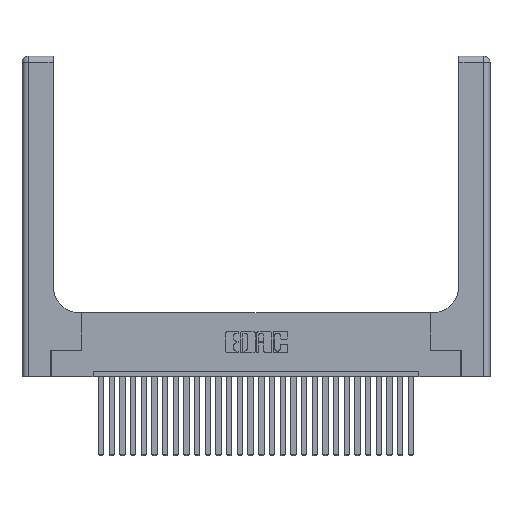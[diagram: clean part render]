
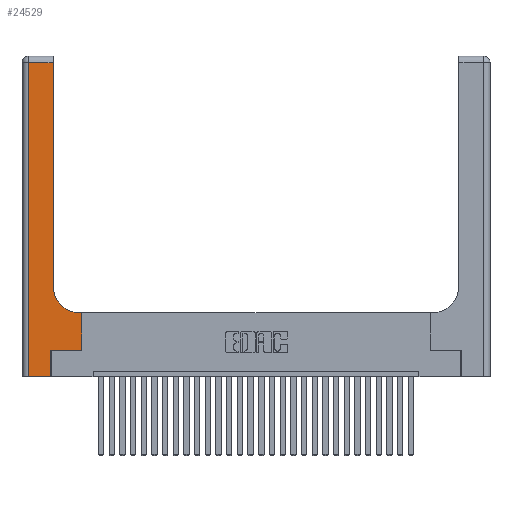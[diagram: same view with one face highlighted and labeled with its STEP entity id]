
A CAD part, top view. The second image highlights one B-rep face of the part: STEP entity #24529.
In plain terms, the highlighted planar face has unit normal (0, 0, 1).
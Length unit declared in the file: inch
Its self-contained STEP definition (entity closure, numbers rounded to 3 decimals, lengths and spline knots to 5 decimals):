
#253 = DIRECTION ( 'NONE',  ( 0., 1., 0. ) ) ;
#806 = LINE ( 'NONE', #20562, #1896 ) ;
#850 = CARTESIAN_POINT ( 'NONE',  ( 0.06, 2.94, 0.37 ) ) ;
#1305 = CARTESIAN_POINT ( 'NONE',  ( 0.5585, 0.25, 0.37 ) ) ;
#1896 = VECTOR ( 'NONE', #9451, 39.37008 ) ;
#2291 = VERTEX_POINT ( 'NONE', #1305 ) ;
#2658 = CARTESIAN_POINT ( 'NONE',  ( 0.2915, 3., 0.37 ) ) ;
#3157 = ORIENTED_EDGE ( 'NONE', *, *, #27383, .T. ) ;
#4992 = VERTEX_POINT ( 'NONE', #10612 ) ;
#5065 = VERTEX_POINT ( 'NONE', #5895 ) ;
#5130 = CARTESIAN_POINT ( 'NONE',  ( 0.269, 0., 0.37 ) ) ;
#5778 = DIRECTION ( 'NONE',  ( 0., 1., 0. ) ) ;
#5825 = EDGE_CURVE ( 'NONE', #5065, #26356, #13908, .T. ) ;
#5841 = FACE_OUTER_BOUND ( 'NONE', #19211, .T. ) ;
#5895 = CARTESIAN_POINT ( 'NONE',  ( 0.06, 0., 0.37 ) ) ;
#6291 = CARTESIAN_POINT ( 'NONE',  ( 0.269, 0.25, 0.37 ) ) ;
#6607 = DIRECTION ( 'NONE',  ( 1., 0., 0. ) ) ;
#7055 = CIRCLE ( 'NONE', #23160, 0.25 ) ;
#7108 = VERTEX_POINT ( 'NONE', #27747 ) ;
#7764 = ORIENTED_EDGE ( 'NONE', *, *, #29153, .T. ) ;
#8100 = CARTESIAN_POINT ( 'NONE',  ( 0.5415, 0.6, 0.37 ) ) ;
#8159 = LINE ( 'NONE', #25982, #11675 ) ;
#8268 = CARTESIAN_POINT ( 'NONE',  ( 0., 3., 0.37 ) ) ;
#9451 = DIRECTION ( 'NONE',  ( 0., -1., 0. ) ) ;
#9475 = EDGE_CURVE ( 'NONE', #4992, #24209, #21478, .T. ) ;
#10612 = CARTESIAN_POINT ( 'NONE',  ( 0.2915, 0.85, 0.37 ) ) ;
#10810 = AXIS2_PLACEMENT_3D ( 'NONE', #8268, #19627, #26710 ) ;
#11675 = VECTOR ( 'NONE', #5778, 39.37008 ) ;
#12214 = LINE ( 'NONE', #17220, #23183 ) ;
#12456 = ORIENTED_EDGE ( 'NONE', *, *, #14858, .T. ) ;
#13082 = ORIENTED_EDGE ( 'NONE', *, *, #5825, .T. ) ;
#13319 = ORIENTED_EDGE ( 'NONE', *, *, #23924, .T. ) ;
#13908 = LINE ( 'NONE', #20807, #17813 ) ;
#14645 = CARTESIAN_POINT ( 'NONE',  ( 0.269, 0., 0.37 ) ) ;
#14767 = ORIENTED_EDGE ( 'NONE', *, *, #26544, .T. ) ;
#14858 = EDGE_CURVE ( 'NONE', #24209, #26318, #20935, .T. ) ;
#15845 = DIRECTION ( 'NONE',  ( 0., 0., -1. ) ) ;
#15990 = DIRECTION ( 'NONE',  ( 1., 0., 0. ) ) ;
#16206 = VERTEX_POINT ( 'NONE', #8100 ) ;
#16241 = LINE ( 'NONE', #5130, #25424 ) ;
#17144 = DIRECTION ( 'NONE',  ( -1., 0., 0. ) ) ;
#17220 = CARTESIAN_POINT ( 'NONE',  ( 0.2915, 0.6, 0.37 ) ) ;
#17341 = CARTESIAN_POINT ( 'NONE',  ( 0., 2.94, 0.37 ) ) ;
#17813 = VECTOR ( 'NONE', #15990, 39.37008 ) ;
#18598 = VERTEX_POINT ( 'NONE', #20325 ) ;
#19211 = EDGE_LOOP ( 'NONE', ( #21373, #12456, #3157, #13082, #27983, #14767, #20211, #13319, #7764 ) ) ;
#19627 = DIRECTION ( 'NONE',  ( 0., 0., -1. ) ) ;
#19844 = DIRECTION ( 'NONE',  ( 1., 0., 0. ) ) ;
#20211 = ORIENTED_EDGE ( 'NONE', *, *, #28252, .T. ) ;
#20325 = CARTESIAN_POINT ( 'NONE',  ( 0.5585, 0.6, 0.37 ) ) ;
#20562 = CARTESIAN_POINT ( 'NONE',  ( 0.06, 3., 0.37 ) ) ;
#20807 = CARTESIAN_POINT ( 'NONE',  ( 0., 0., 0.37 ) ) ;
#20935 = LINE ( 'NONE', #17341, #24841 ) ;
#21373 = ORIENTED_EDGE ( 'NONE', *, *, #9475, .T. ) ;
#21478 = LINE ( 'NONE', #2658, #25752 ) ;
#21795 = PLANE ( 'NONE',  #10810 ) ;
#21835 = EDGE_CURVE ( 'NONE', #26356, #7108, #16241, .T. ) ;
#22596 = CARTESIAN_POINT ( 'NONE',  ( 0.2915, 2.94, 0.37 ) ) ;
#22920 = DIRECTION ( 'NONE',  ( 0., 1., 0. ) ) ;
#23160 = AXIS2_PLACEMENT_3D ( 'NONE', #24453, #15845, #6607 ) ;
#23183 = VECTOR ( 'NONE', #26475, 39.37008 ) ;
#23924 = EDGE_CURVE ( 'NONE', #18598, #16206, #12214, .T. ) ;
#24128 = VECTOR ( 'NONE', #19844, 39.37008 ) ;
#24209 = VERTEX_POINT ( 'NONE', #22596 ) ;
#24453 = CARTESIAN_POINT ( 'NONE',  ( 0.5415, 0.85, 0.37 ) ) ;
#24529 = ADVANCED_FACE ( 'NONE', ( #5841 ), #21795, .F. ) ;
#24841 = VECTOR ( 'NONE', #17144, 39.37008 ) ;
#25424 = VECTOR ( 'NONE', #253, 39.37008 ) ;
#25752 = VECTOR ( 'NONE', #22920, 39.37008 ) ;
#25982 = CARTESIAN_POINT ( 'NONE',  ( 0.5585, 0.25, 0.37 ) ) ;
#26318 = VERTEX_POINT ( 'NONE', #850 ) ;
#26356 = VERTEX_POINT ( 'NONE', #14645 ) ;
#26475 = DIRECTION ( 'NONE',  ( -1., 0., 0. ) ) ;
#26544 = EDGE_CURVE ( 'NONE', #7108, #2291, #26916, .T. ) ;
#26710 = DIRECTION ( 'NONE',  ( -1., 0., 0. ) ) ;
#26916 = LINE ( 'NONE', #6291, #24128 ) ;
#27383 = EDGE_CURVE ( 'NONE', #26318, #5065, #806, .T. ) ;
#27747 = CARTESIAN_POINT ( 'NONE',  ( 0.269, 0.25, 0.37 ) ) ;
#27983 = ORIENTED_EDGE ( 'NONE', *, *, #21835, .T. ) ;
#28252 = EDGE_CURVE ( 'NONE', #2291, #18598, #8159, .T. ) ;
#29153 = EDGE_CURVE ( 'NONE', #16206, #4992, #7055, .T. ) ;
